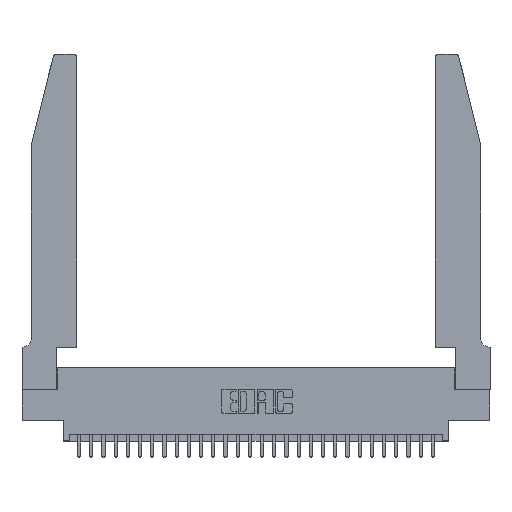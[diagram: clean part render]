
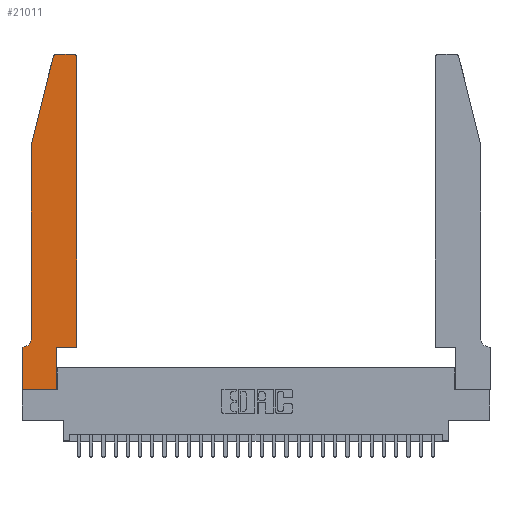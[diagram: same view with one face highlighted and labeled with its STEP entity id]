
A CAD part, top view. The second image highlights one B-rep face of the part: STEP entity #21011.
In plain terms, the highlighted planar face has unit normal (0, 0, 1).
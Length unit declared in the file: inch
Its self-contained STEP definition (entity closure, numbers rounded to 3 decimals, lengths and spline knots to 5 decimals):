
#93 = EDGE_CURVE ( 'NONE', #26209, #19957, #29565, .T. ) ;
#302 = DIRECTION ( 'NONE',  ( 1., 0., 0. ) ) ;
#1309 = ORIENTED_EDGE ( 'NONE', *, *, #93, .T. ) ;
#1360 = LINE ( 'NONE', #19968, #10781 ) ;
#1671 = VERTEX_POINT ( 'NONE', #15941 ) ;
#1765 = LINE ( 'NONE', #18382, #21768 ) ;
#1827 = CARTESIAN_POINT ( 'NONE',  ( 0., 0.35, 0.37 ) ) ;
#2237 = VERTEX_POINT ( 'NONE', #18124 ) ;
#2295 = EDGE_CURVE ( 'NONE', #19141, #26209, #23618, .T. ) ;
#2592 = CARTESIAN_POINT ( 'NONE',  ( 0.284, 2.72, 0.37 ) ) ;
#3646 = VERTEX_POINT ( 'NONE', #1827 ) ;
#3758 = EDGE_LOOP ( 'NONE', ( #5804, #10115, #1309, #9953, #8366, #14596, #28471, #25736, #21584, #17012, #25495, #7958 ) ) ;
#4873 = PLANE ( 'NONE',  #6132 ) ;
#4978 = DIRECTION ( 'NONE',  ( 1., 0., 0. ) ) ;
#4996 = DIRECTION ( 'NONE',  ( 0., 0., 1. ) ) ;
#5520 = DIRECTION ( 'NONE',  ( 0., 1., 0. ) ) ;
#5804 = ORIENTED_EDGE ( 'NONE', *, *, #26029, .T. ) ;
#6132 = AXIS2_PLACEMENT_3D ( 'NONE', #26098, #9452, #4978 ) ;
#6680 = VECTOR ( 'NONE', #20913, 39.37008 ) ;
#7055 = AXIS2_PLACEMENT_3D ( 'NONE', #2592, #4996, #18803 ) ;
#7139 = VECTOR ( 'NONE', #24594, 39.37008 ) ;
#7406 = DIRECTION ( 'NONE',  ( 0., 0., 1. ) ) ;
#7713 = VECTOR ( 'NONE', #302, 39.37008 ) ;
#7902 = EDGE_CURVE ( 'NONE', #16540, #27953, #23380, .T. ) ;
#7958 = ORIENTED_EDGE ( 'NONE', *, *, #19965, .T. ) ;
#8361 = CARTESIAN_POINT ( 'NONE',  ( 0.0055, 0.42, 0.37 ) ) ;
#8366 = ORIENTED_EDGE ( 'NONE', *, *, #7902, .T. ) ;
#9335 = CARTESIAN_POINT ( 'NONE',  ( 0.4505, 0.35, 0.37 ) ) ;
#9452 = DIRECTION ( 'NONE',  ( 0., 0., 1. ) ) ;
#9716 = DIRECTION ( 'NONE',  ( 1., 0., 0. ) ) ;
#9893 = CARTESIAN_POINT ( 'NONE',  ( 0.0055, 0.35, 0.37 ) ) ;
#9953 = ORIENTED_EDGE ( 'NONE', *, *, #23756, .T. ) ;
#9999 = AXIS2_PLACEMENT_3D ( 'NONE', #14526, #7406, #9716 ) ;
#10115 = ORIENTED_EDGE ( 'NONE', *, *, #2295, .T. ) ;
#10546 = LINE ( 'NONE', #20313, #22173 ) ;
#10548 = CARTESIAN_POINT ( 'NONE',  ( 0.0755, 0.42, 0.37 ) ) ;
#10781 = VECTOR ( 'NONE', #22316, 39.37008 ) ;
#11502 = DIRECTION ( 'NONE',  ( 0., 1., 0. ) ) ;
#11870 = LINE ( 'NONE', #17531, #7139 ) ;
#12393 = AXIS2_PLACEMENT_3D ( 'NONE', #8361, #25312, #20160 ) ;
#12481 = LINE ( 'NONE', #14586, #27686 ) ;
#13607 = EDGE_CURVE ( 'NONE', #15192, #18468, #1765, .T. ) ;
#14526 = CARTESIAN_POINT ( 'NONE',  ( 0.4205, 2.72, 0.37 ) ) ;
#14586 = CARTESIAN_POINT ( 'NONE',  ( 0.4505, 0.35, 0.37 ) ) ;
#14596 = ORIENTED_EDGE ( 'NONE', *, *, #23722, .T. ) ;
#14673 = LINE ( 'NONE', #27906, #6680 ) ;
#14836 = CARTESIAN_POINT ( 'NONE',  ( 0.0755, 2., 0.37 ) ) ;
#15192 = VERTEX_POINT ( 'NONE', #29301 ) ;
#15212 = CARTESIAN_POINT ( 'NONE',  ( 0.4505, 0.35, 0.37 ) ) ;
#15579 = CARTESIAN_POINT ( 'NONE',  ( 0.0755, 0.35, 0.37 ) ) ;
#15770 = CARTESIAN_POINT ( 'NONE',  ( 0.0755, 2., 0.37 ) ) ;
#15941 = CARTESIAN_POINT ( 'NONE',  ( 0.4505, 2.72, 0.37 ) ) ;
#16540 = VERTEX_POINT ( 'NONE', #10548 ) ;
#16891 = EDGE_CURVE ( 'NONE', #18468, #27618, #18606, .T. ) ;
#16957 = CIRCLE ( 'NONE', #9999, 0.03 ) ;
#17012 = ORIENTED_EDGE ( 'NONE', *, *, #16891, .T. ) ;
#17531 = CARTESIAN_POINT ( 'NONE',  ( 0., 0., 0.37 ) ) ;
#17838 = CARTESIAN_POINT ( 'NONE',  ( 0.4205, 2.75, 0.37 ) ) ;
#18124 = CARTESIAN_POINT ( 'NONE',  ( 0., 0., 0.37 ) ) ;
#18127 = VERTEX_POINT ( 'NONE', #17838 ) ;
#18382 = CARTESIAN_POINT ( 'NONE',  ( 0.2865, 0.35, 0.37 ) ) ;
#18468 = VERTEX_POINT ( 'NONE', #28063 ) ;
#18606 = LINE ( 'NONE', #9335, #7713 ) ;
#18803 = DIRECTION ( 'NONE',  ( 1., 0., 0. ) ) ;
#19141 = VERTEX_POINT ( 'NONE', #23104 ) ;
#19610 = VECTOR ( 'NONE', #27417, 39.37008 ) ;
#19957 = VERTEX_POINT ( 'NONE', #14836 ) ;
#19965 = EDGE_CURVE ( 'NONE', #1671, #18127, #16957, .T. ) ;
#19968 = CARTESIAN_POINT ( 'NONE',  ( 0.2605, 2.75, 0.37 ) ) ;
#20160 = DIRECTION ( 'NONE',  ( -1., 0., 0. ) ) ;
#20313 = CARTESIAN_POINT ( 'NONE',  ( 0.0755, 2., 0.37 ) ) ;
#20647 = EDGE_CURVE ( 'NONE', #3646, #2237, #11870, .T. ) ;
#20913 = DIRECTION ( 'NONE',  ( 1., 0., 0. ) ) ;
#21011 = ADVANCED_FACE ( 'NONE', ( #25964 ), #4873, .T. ) ;
#21584 = ORIENTED_EDGE ( 'NONE', *, *, #13607, .T. ) ;
#21768 = VECTOR ( 'NONE', #11502, 39.37008 ) ;
#22131 = EDGE_CURVE ( 'NONE', #2237, #15192, #14673, .T. ) ;
#22173 = VECTOR ( 'NONE', #29559, 39.37008 ) ;
#22316 = DIRECTION ( 'NONE',  ( -1., 0., 0. ) ) ;
#23104 = CARTESIAN_POINT ( 'NONE',  ( 0.284, 2.75, 0.37 ) ) ;
#23328 = CARTESIAN_POINT ( 'NONE',  ( 0.25487, 2.72718, 0.37 ) ) ;
#23380 = CIRCLE ( 'NONE', #12393, 0.07 ) ;
#23618 = CIRCLE ( 'NONE', #7055, 0.03 ) ;
#23722 = EDGE_CURVE ( 'NONE', #27953, #3646, #24330, .T. ) ;
#23756 = EDGE_CURVE ( 'NONE', #19957, #16540, #10546, .T. ) ;
#24330 = LINE ( 'NONE', #15579, #19610 ) ;
#24594 = DIRECTION ( 'NONE',  ( 0., -1., 0. ) ) ;
#25312 = DIRECTION ( 'NONE',  ( 0., 0., -1. ) ) ;
#25495 = ORIENTED_EDGE ( 'NONE', *, *, #27970, .T. ) ;
#25736 = ORIENTED_EDGE ( 'NONE', *, *, #22131, .T. ) ;
#25964 = FACE_OUTER_BOUND ( 'NONE', #3758, .T. ) ;
#26029 = EDGE_CURVE ( 'NONE', #18127, #19141, #1360, .T. ) ;
#26098 = CARTESIAN_POINT ( 'NONE',  ( 0., 0.35, 0.37 ) ) ;
#26209 = VERTEX_POINT ( 'NONE', #23328 ) ;
#26989 = DIRECTION ( 'NONE',  ( -0.239, -0.971, 0. ) ) ;
#27003 = VECTOR ( 'NONE', #26989, 39.37008 ) ;
#27417 = DIRECTION ( 'NONE',  ( -1., 0., 0. ) ) ;
#27618 = VERTEX_POINT ( 'NONE', #15212 ) ;
#27686 = VECTOR ( 'NONE', #5520, 39.37008 ) ;
#27906 = CARTESIAN_POINT ( 'NONE',  ( 0., 0., 0.37 ) ) ;
#27953 = VERTEX_POINT ( 'NONE', #9893 ) ;
#27970 = EDGE_CURVE ( 'NONE', #27618, #1671, #12481, .T. ) ;
#28063 = CARTESIAN_POINT ( 'NONE',  ( 0.2865, 0.35, 0.37 ) ) ;
#28471 = ORIENTED_EDGE ( 'NONE', *, *, #20647, .T. ) ;
#29301 = CARTESIAN_POINT ( 'NONE',  ( 0.2865, 0., 0.37 ) ) ;
#29559 = DIRECTION ( 'NONE',  ( 0., -1., 0. ) ) ;
#29565 = LINE ( 'NONE', #15770, #27003 ) ;
